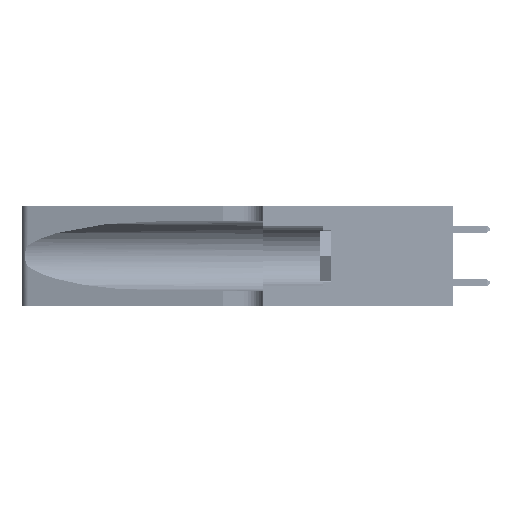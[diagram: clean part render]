
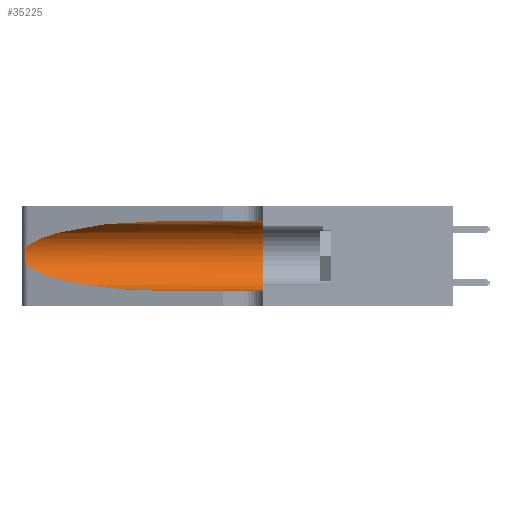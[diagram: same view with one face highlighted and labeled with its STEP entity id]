
A CAD part, left-side view. The second image highlights one B-rep face of the part: STEP entity #35225.
In plain terms, the highlighted cylindrical face has radius 3.308 mm (diameter 6.617 mm), a partial arc.
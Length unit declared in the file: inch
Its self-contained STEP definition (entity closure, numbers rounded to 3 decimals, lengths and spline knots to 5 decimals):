
#553 = CARTESIAN_POINT ( 'NONE',  ( 0.25555, 1.22993, 0.14849 ) ) ;
#722 = DIRECTION ( 'NONE',  ( 0., -1., 0. ) ) ;
#1702 =( BOUNDED_CURVE ( )  B_SPLINE_CURVE ( 3, ( #30163, #3190, #14960, #41521 ),
 .UNSPECIFIED., .F., .F. ) 
 B_SPLINE_CURVE_WITH_KNOTS ( ( 4, 4 ),
 ( 3.44316, 4.71239 ),
 .UNSPECIFIED. ) 
 CURVE ( )  GEOMETRIC_REPRESENTATION_ITEM ( )  RATIONAL_B_SPLINE_CURVE ( ( 1., 0.87, 0.87, 1. ) ) 
 REPRESENTATION_ITEM ( '' )  );
#1910 = CIRCLE ( 'NONE', #26856, 0.13025 ) ;
#2696 = FACE_OUTER_BOUND ( 'NONE', #45842, .T. ) ;
#3190 = CARTESIAN_POINT ( 'NONE',  ( 0.2373, 1.15595, 0.08982 ) ) ;
#3670 = ORIENTED_EDGE ( 'NONE', *, *, #43315, .T. ) ;
#5907 = ORIENTED_EDGE ( 'NONE', *, *, #22353, .F. ) ;
#8265 = CARTESIAN_POINT ( 'NONE',  ( 0.25787, 1.23484, 0.2124 ) ) ;
#9729 = CARTESIAN_POINT ( 'NONE',  ( 0.25487, 1.22718, 0.14631 ) ) ;
#12197 = CARTESIAN_POINT ( 'NONE',  ( 0.26018, 1.23835, 0.19895 ) ) ;
#14651 = VERTEX_POINT ( 'NONE', #16182 ) ;
#14960 = CARTESIAN_POINT ( 'NONE',  ( 0.18966, 0.96281, 0.05475 ) ) ;
#16117 = CARTESIAN_POINT ( 'NONE',  ( 0.26075, 1.23896, 0.178 ) ) ;
#16182 = CARTESIAN_POINT ( 'NONE',  ( 0.1305, 0.35, 0.05475 ) ) ;
#16240 = ORIENTED_EDGE ( 'NONE', *, *, #47708, .T. ) ;
#16347 = DIRECTION ( 'NONE',  ( 0., 1., 0. ) ) ;
#16810 = CARTESIAN_POINT ( 'NONE',  ( 0.1305, 0.72297, 0.05475 ) ) ;
#17384 = CARTESIAN_POINT ( 'NONE',  ( 0.1305, 0.35, 0.31525 ) ) ;
#19193 = LINE ( 'NONE', #27789, #20392 ) ;
#19291 = VERTEX_POINT ( 'NONE', #22837 ) ;
#19834 =( BOUNDED_CURVE ( )  B_SPLINE_CURVE ( 3, ( #45332, #34111, #22869, #49313 ),
 .UNSPECIFIED., .F., .F. ) 
 B_SPLINE_CURVE_WITH_KNOTS ( ( 4, 4 ),
 ( 1.5708, 2.84003 ),
 .UNSPECIFIED. ) 
 CURVE ( )  GEOMETRIC_REPRESENTATION_ITEM ( )  RATIONAL_B_SPLINE_CURVE ( ( 1., 0.87, 0.87, 1. ) ) 
 REPRESENTATION_ITEM ( '' )  );
#19863 = CARTESIAN_POINT ( 'NONE',  ( 0.25555, 1.22994, 0.2215 ) ) ;
#20019 = CARTESIAN_POINT ( 'NONE',  ( 0.25856, 1.23593, 0.16098 ) ) ;
#20392 = VECTOR ( 'NONE', #722, 39.37008 ) ;
#20440 = AXIS2_PLACEMENT_3D ( 'NONE', #30475, #23037, #26871 ) ;
#21424 = EDGE_CURVE ( 'NONE', #46424, #46562, #46165, .T. ) ;
#22353 = EDGE_CURVE ( 'NONE', #19291, #44959, #25867, .T. ) ;
#22837 = CARTESIAN_POINT ( 'NONE',  ( 0.1305, 0.72297, 0.31525 ) ) ;
#22869 = CARTESIAN_POINT ( 'NONE',  ( 0.2373, 1.15595, 0.28018 ) ) ;
#23037 = DIRECTION ( 'NONE',  ( 0., -1., 0. ) ) ;
#23835 = CARTESIAN_POINT ( 'NONE',  ( 0.25639, 1.23186, 0.15144 ) ) ;
#24807 = ORIENTED_EDGE ( 'NONE', *, *, #36804, .F. ) ;
#25867 = LINE ( 'NONE', #32972, #27033 ) ;
#26856 = AXIS2_PLACEMENT_3D ( 'NONE', #39080, #16347, #42875 ) ;
#26871 = DIRECTION ( 'NONE',  ( 0., 0., -1. ) ) ;
#27033 = VECTOR ( 'NONE', #36762, 39.37008 ) ;
#27497 = CARTESIAN_POINT ( 'NONE',  ( 0.25639, 1.23184, 0.21858 ) ) ;
#27648 = CARTESIAN_POINT ( 'NONE',  ( 0.25487, 1.22718, 0.14631 ) ) ;
#27789 = CARTESIAN_POINT ( 'NONE',  ( 0.1305, 1.61858, 0.05475 ) ) ;
#30163 = CARTESIAN_POINT ( 'NONE',  ( 0.25487, 1.22718, 0.14631 ) ) ;
#30475 = CARTESIAN_POINT ( 'NONE',  ( 0.1305, 1.61858, 0.185 ) ) ;
#30722 = VERTEX_POINT ( 'NONE', #16810 ) ;
#31266 = CARTESIAN_POINT ( 'NONE',  ( 0.25487, 1.22718, 0.22369 ) ) ;
#32972 = CARTESIAN_POINT ( 'NONE',  ( 0.1305, 1.61858, 0.31525 ) ) ;
#34111 = CARTESIAN_POINT ( 'NONE',  ( 0.18966, 0.96281, 0.31525 ) ) ;
#35054 = CARTESIAN_POINT ( 'NONE',  ( 0.25854, 1.2359, 0.20912 ) ) ;
#35225 = ADVANCED_FACE ( 'NONE', ( #2696 ), #42228, .F. ) ;
#35971 = ORIENTED_EDGE ( 'NONE', *, *, #21424, .T. ) ;
#36762 = DIRECTION ( 'NONE',  ( 0., -1., 0. ) ) ;
#36804 = EDGE_CURVE ( 'NONE', #44959, #14651, #1910, .T. ) ;
#37305 = ORIENTED_EDGE ( 'NONE', *, *, #39453, .T. ) ;
#38843 = CARTESIAN_POINT ( 'NONE',  ( 0.26075, 1.23896, 0.19203 ) ) ;
#39080 = CARTESIAN_POINT ( 'NONE',  ( 0.1305, 0.35, 0.185 ) ) ;
#39453 = EDGE_CURVE ( 'NONE', #19291, #46424, #19834, .T. ) ;
#41521 = CARTESIAN_POINT ( 'NONE',  ( 0.1305, 0.72297, 0.05475 ) ) ;
#42228 = CYLINDRICAL_SURFACE ( 'NONE', #20440, 0.13025 ) ;
#42643 = CARTESIAN_POINT ( 'NONE',  ( 0.26017, 1.23833, 0.17102 ) ) ;
#42875 = DIRECTION ( 'NONE',  ( 0., 0., 1. ) ) ;
#43315 = EDGE_CURVE ( 'NONE', #46562, #30722, #1702, .T. ) ;
#44959 = VERTEX_POINT ( 'NONE', #17384 ) ;
#45332 = CARTESIAN_POINT ( 'NONE',  ( 0.1305, 0.72297, 0.31525 ) ) ;
#45842 = EDGE_LOOP ( 'NONE', ( #37305, #35971, #3670, #16240, #24807, #5907 ) ) ;
#46165 = B_SPLINE_CURVE_WITH_KNOTS ( 'NONE', 3,
 ( #31266, #19863, #27497, #8265, #35054, #12197, #38843, #16117, #42643, #20019, #46444, #23835, #553, #27648 ),
 .UNSPECIFIED., .F., .F.,
 ( 4, 2, 2, 2, 2, 2, 4 ),
 ( 0., 0.00027, 0.00053, 0.00107, 0.0016, 0.00187, 0.00214 ),
 .UNSPECIFIED. ) ;
#46424 = VERTEX_POINT ( 'NONE', #47222 ) ;
#46444 = CARTESIAN_POINT ( 'NONE',  ( 0.25789, 1.23486, 0.15765 ) ) ;
#46562 = VERTEX_POINT ( 'NONE', #9729 ) ;
#47222 = CARTESIAN_POINT ( 'NONE',  ( 0.25487, 1.22718, 0.22369 ) ) ;
#47708 = EDGE_CURVE ( 'NONE', #30722, #14651, #19193, .T. ) ;
#49313 = CARTESIAN_POINT ( 'NONE',  ( 0.25487, 1.22718, 0.22369 ) ) ;
